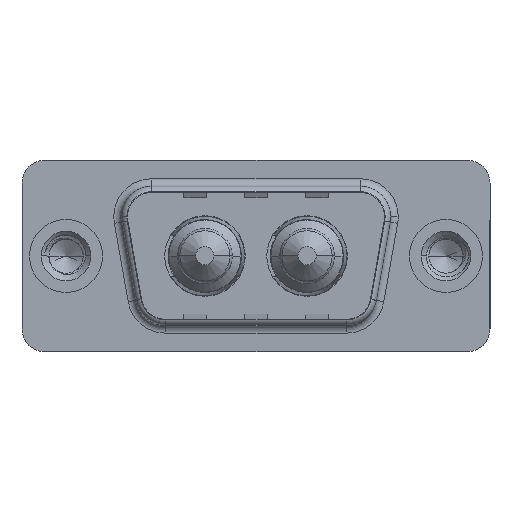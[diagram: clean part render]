
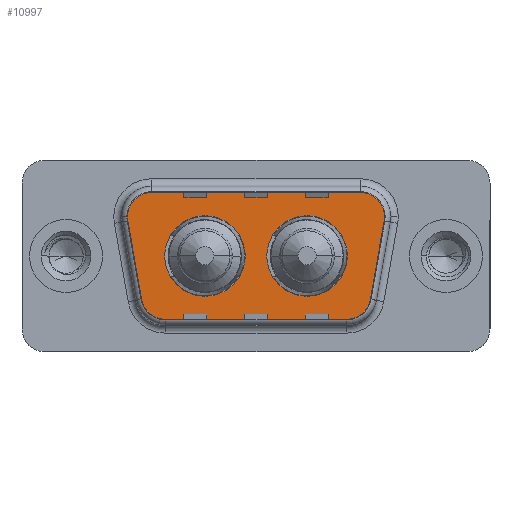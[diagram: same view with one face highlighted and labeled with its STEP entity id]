
A CAD part, top view. The second image highlights one B-rep face of the part: STEP entity #10997.
In plain terms, the highlighted planar face has unit normal (0, 0, 1).
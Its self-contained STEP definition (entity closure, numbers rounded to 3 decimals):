
#28 = AXIS2_PLACEMENT_3D ( 'NONE', #11418, #16136, #16488 ) ;
#136 = DIRECTION ( 'NONE',  ( 1., 0., 0. ) ) ;
#182 = DIRECTION ( 'NONE',  ( 0., 0., 1. ) ) ;
#240 = CARTESIAN_POINT ( 'NONE',  ( 9.14, 0., 0. ) ) ;
#304 = CARTESIAN_POINT ( 'NONE',  ( 11.79, 0., 0. ) ) ;
#706 = CARTESIAN_POINT ( 'NONE',  ( 18.541, -2.9, 0. ) ) ;
#716 = VERTEX_POINT ( 'NONE', #2600 ) ;
#752 = PLANE ( 'NONE',  #10680 ) ;
#861 = FACE_BOUND ( 'NONE', #10428, .T. ) ;
#1129 = EDGE_CURVE ( 'NONE', #3359, #14123, #5185, .T. ) ;
#1335 = EDGE_CURVE ( 'NONE', #14123, #3359, #9990, .T. ) ;
#1551 = CIRCLE ( 'NONE', #15464, 2. ) ;
#1578 = DIRECTION ( 'NONE',  ( 0.174, -0.985, 0. ) ) ;
#1674 = LINE ( 'NONE', #4433, #11470 ) ;
#1709 = DIRECTION ( 'NONE',  ( 0., 0., 1. ) ) ;
#1914 = CARTESIAN_POINT ( 'NONE',  ( 3.466, 2.553, 0. ) ) ;
#1973 = CARTESIAN_POINT ( 'NONE',  ( 6.459, -4.9, 0. ) ) ;
#2017 = DIRECTION ( 'NONE',  ( 1., 0., 0. ) ) ;
#2100 = ORIENTED_EDGE ( 'NONE', *, *, #7287, .F. ) ;
#2186 = DIRECTION ( 'NONE',  ( 0., 0., 1. ) ) ;
#2193 = CARTESIAN_POINT ( 'NONE',  ( 18.541, -2.9, 0. ) ) ;
#2461 = ORIENTED_EDGE ( 'NONE', *, *, #3976, .T. ) ;
#2474 = VERTEX_POINT ( 'NONE', #4609 ) ;
#2521 = AXIS2_PLACEMENT_3D ( 'NONE', #4147, #13204, #5457 ) ;
#2600 = CARTESIAN_POINT ( 'NONE',  ( 18.541, -4.9, 0. ) ) ;
#2649 = CARTESIAN_POINT ( 'NONE',  ( 21.564, 2.9, 0. ) ) ;
#3004 = AXIS2_PLACEMENT_3D ( 'NONE', #240, #182, #136 ) ;
#3240 = CARTESIAN_POINT ( 'NONE',  ( 13.21, 0., 0. ) ) ;
#3359 = VERTEX_POINT ( 'NONE', #7092 ) ;
#3409 = CARTESIAN_POINT ( 'NONE',  ( 6.459, -4.9, 0. ) ) ;
#3438 = DIRECTION ( 'NONE',  ( 1., 0., 0. ) ) ;
#3457 = DIRECTION ( 'NONE',  ( 1., 0., 0. ) ) ;
#3472 = EDGE_CURVE ( 'NONE', #6831, #12995, #16606, .T. ) ;
#3759 = ORIENTED_EDGE ( 'NONE', *, *, #12597, .F. ) ;
#3976 = EDGE_CURVE ( 'NONE', #14890, #14078, #1551, .T. ) ;
#4147 = CARTESIAN_POINT ( 'NONE',  ( 5.436, 2.9, 0. ) ) ;
#4184 = VERTEX_POINT ( 'NONE', #14589 ) ;
#4268 = VECTOR ( 'NONE', #3457, 1000. ) ;
#4433 = CARTESIAN_POINT ( 'NONE',  ( 21.534, 2.553, 0. ) ) ;
#4609 = CARTESIAN_POINT ( 'NONE',  ( 20.511, -3.247, 0. ) ) ;
#4650 = LINE ( 'NONE', #9418, #7692 ) ;
#4686 = CIRCLE ( 'NONE', #2521, 2. ) ;
#4953 = ORIENTED_EDGE ( 'NONE', *, *, #1129, .F. ) ;
#5040 = ORIENTED_EDGE ( 'NONE', *, *, #15319, .T. ) ;
#5185 = CIRCLE ( 'NONE', #14112, 2.65 ) ;
#5354 = ORIENTED_EDGE ( 'NONE', *, *, #9016, .T. ) ;
#5457 = DIRECTION ( 'NONE',  ( 1., 0., 0. ) ) ;
#5671 = DIRECTION ( 'NONE',  ( 0., 0., 1. ) ) ;
#5775 = ORIENTED_EDGE ( 'NONE', *, *, #3472, .T. ) ;
#6138 = DIRECTION ( 'NONE',  ( 1., 0., 0. ) ) ;
#6520 = CIRCLE ( 'NONE', #3004, 2.65 ) ;
#6831 = VERTEX_POINT ( 'NONE', #7464 ) ;
#6842 = ORIENTED_EDGE ( 'NONE', *, *, #1335, .F. ) ;
#6981 = CARTESIAN_POINT ( 'NONE',  ( 19.564, 2.9, 0. ) ) ;
#6985 = VERTEX_POINT ( 'NONE', #1914 ) ;
#7092 = CARTESIAN_POINT ( 'NONE',  ( 18.51, 0., 0. ) ) ;
#7268 = VECTOR ( 'NONE', #1578, 1000. ) ;
#7287 = EDGE_CURVE ( 'NONE', #4184, #8030, #6520, .T. ) ;
#7326 = ORIENTED_EDGE ( 'NONE', *, *, #13946, .T. ) ;
#7343 = CIRCLE ( 'NONE', #14789, 2.65 ) ;
#7464 = CARTESIAN_POINT ( 'NONE',  ( 21.534, 2.553, 0. ) ) ;
#7601 = VERTEX_POINT ( 'NONE', #12970 ) ;
#7609 = FACE_BOUND ( 'NONE', #14279, .T. ) ;
#7692 = VECTOR ( 'NONE', #8090, 1000. ) ;
#7694 = LINE ( 'NONE', #3409, #4268 ) ;
#7752 = ORIENTED_EDGE ( 'NONE', *, *, #9731, .T. ) ;
#8030 = VERTEX_POINT ( 'NONE', #304 ) ;
#8090 = DIRECTION ( 'NONE',  ( -1., 0., 0. ) ) ;
#8176 = ORIENTED_EDGE ( 'NONE', *, *, #8375, .T. ) ;
#8260 = DIRECTION ( 'NONE',  ( -1., 0., 0. ) ) ;
#8375 = EDGE_CURVE ( 'NONE', #14078, #716, #7694, .T. ) ;
#9016 = EDGE_CURVE ( 'NONE', #6985, #14890, #14601, .T. ) ;
#9175 = DIRECTION ( 'NONE',  ( 1., 0., 0. ) ) ;
#9384 = AXIS2_PLACEMENT_3D ( 'NONE', #16366, #1709, #6138 ) ;
#9418 = CARTESIAN_POINT ( 'NONE',  ( 5.436, 4.9, 0. ) ) ;
#9651 = DIRECTION ( 'NONE',  ( 0., 0., 1. ) ) ;
#9731 = EDGE_CURVE ( 'NONE', #2474, #6831, #1674, .T. ) ;
#9990 = CIRCLE ( 'NONE', #9384, 2.65 ) ;
#10083 = AXIS2_PLACEMENT_3D ( 'NONE', #2193, #11118, #3438 ) ;
#10428 = EDGE_LOOP ( 'NONE', ( #3759, #2100 ) ) ;
#10620 = FACE_OUTER_BOUND ( 'NONE', #16484, .T. ) ;
#10680 = AXIS2_PLACEMENT_3D ( 'NONE', #706, #9651, #2017 ) ;
#10861 = DIRECTION ( 'NONE',  ( 0., 0., 1. ) ) ;
#10997 = ADVANCED_FACE ( 'NONE', ( #7609, #861, #10620 ), #752, .T. ) ;
#11103 = CARTESIAN_POINT ( 'NONE',  ( 4.489, -3.247, 0. ) ) ;
#11118 = DIRECTION ( 'NONE',  ( 0., 0., 1. ) ) ;
#11376 = CIRCLE ( 'NONE', #10083, 2. ) ;
#11418 = CARTESIAN_POINT ( 'NONE',  ( 19.564, 2.9, 0. ) ) ;
#11470 = VECTOR ( 'NONE', #13521, 1000. ) ;
#11851 = ORIENTED_EDGE ( 'NONE', *, *, #12750, .T. ) ;
#12189 = EDGE_CURVE ( 'NONE', #12995, #7601, #14498, .T. ) ;
#12597 = EDGE_CURVE ( 'NONE', #8030, #4184, #7343, .T. ) ;
#12750 = EDGE_CURVE ( 'NONE', #716, #2474, #11376, .T. ) ;
#12930 = ORIENTED_EDGE ( 'NONE', *, *, #12189, .T. ) ;
#12970 = CARTESIAN_POINT ( 'NONE',  ( 19.564, 4.9, 0. ) ) ;
#12995 = VERTEX_POINT ( 'NONE', #2649 ) ;
#13204 = DIRECTION ( 'NONE',  ( 0., 0., 1. ) ) ;
#13449 = CARTESIAN_POINT ( 'NONE',  ( 9.14, 0., 0. ) ) ;
#13521 = DIRECTION ( 'NONE',  ( 0.174, 0.985, 0. ) ) ;
#13946 = EDGE_CURVE ( 'NONE', #16448, #6985, #4686, .T. ) ;
#14078 = VERTEX_POINT ( 'NONE', #1973 ) ;
#14112 = AXIS2_PLACEMENT_3D ( 'NONE', #16468, #10861, #9175 ) ;
#14123 = VERTEX_POINT ( 'NONE', #3240 ) ;
#14279 = EDGE_LOOP ( 'NONE', ( #4953, #6842 ) ) ;
#14414 = CARTESIAN_POINT ( 'NONE',  ( 3.466, 2.553, 0. ) ) ;
#14498 = CIRCLE ( 'NONE', #15098, 2. ) ;
#14589 = CARTESIAN_POINT ( 'NONE',  ( 6.49, 0., 0. ) ) ;
#14601 = LINE ( 'NONE', #14414, #7268 ) ;
#14749 = DIRECTION ( 'NONE',  ( 1., 0., 0. ) ) ;
#14789 = AXIS2_PLACEMENT_3D ( 'NONE', #13449, #5671, #14749 ) ;
#14822 = CARTESIAN_POINT ( 'NONE',  ( 5.436, 4.9, 0. ) ) ;
#14890 = VERTEX_POINT ( 'NONE', #11103 ) ;
#15098 = AXIS2_PLACEMENT_3D ( 'NONE', #6981, #15996, #8260 ) ;
#15319 = EDGE_CURVE ( 'NONE', #7601, #16448, #4650, .T. ) ;
#15464 = AXIS2_PLACEMENT_3D ( 'NONE', #15940, #2186, #15887 ) ;
#15887 = DIRECTION ( 'NONE',  ( -1., 0., 0. ) ) ;
#15940 = CARTESIAN_POINT ( 'NONE',  ( 6.459, -2.9, 0. ) ) ;
#15996 = DIRECTION ( 'NONE',  ( 0., 0., 1. ) ) ;
#16136 = DIRECTION ( 'NONE',  ( 0., 0., 1. ) ) ;
#16366 = CARTESIAN_POINT ( 'NONE',  ( 15.86, 0., 0. ) ) ;
#16448 = VERTEX_POINT ( 'NONE', #14822 ) ;
#16468 = CARTESIAN_POINT ( 'NONE',  ( 15.86, 0., 0. ) ) ;
#16484 = EDGE_LOOP ( 'NONE', ( #11851, #7752, #5775, #12930, #5040, #7326, #5354, #2461, #8176 ) ) ;
#16488 = DIRECTION ( 'NONE',  ( -1., 0., 0. ) ) ;
#16606 = CIRCLE ( 'NONE', #28, 2. ) ;
